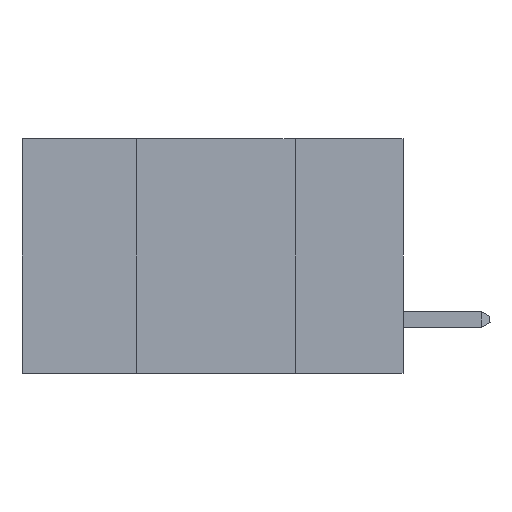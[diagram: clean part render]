
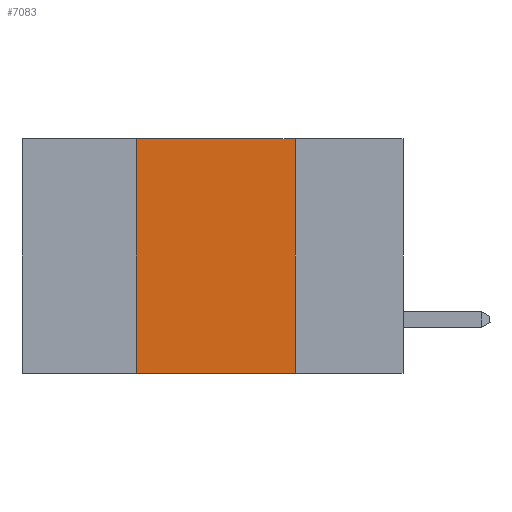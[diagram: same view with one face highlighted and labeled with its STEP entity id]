
A CAD part, left-side view. The second image highlights one B-rep face of the part: STEP entity #7083.
In plain terms, the highlighted planar face has unit normal (-1, 0, 0).
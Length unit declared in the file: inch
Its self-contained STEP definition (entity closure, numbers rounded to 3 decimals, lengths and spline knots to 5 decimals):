
#1003 = VERTEX_POINT ( 'NONE', #19001 ) ;
#2471 = EDGE_CURVE ( 'NONE', #4461, #5090, #20373, .T. ) ;
#3396 = EDGE_LOOP ( 'NONE', ( #16093, #5084, #22104, #19474 ) ) ;
#3500 = FACE_OUTER_BOUND ( 'NONE', #3396, .T. ) ;
#4435 = VECTOR ( 'NONE', #12951, 39.37008 ) ;
#4461 = VERTEX_POINT ( 'NONE', #22385 ) ;
#4968 = CARTESIAN_POINT ( 'NONE',  ( 0., 0.6, 0. ) ) ;
#5084 = ORIENTED_EDGE ( 'NONE', *, *, #2471, .F. ) ;
#5090 = VERTEX_POINT ( 'NONE', #24746 ) ;
#5324 = DIRECTION ( 'NONE',  ( 1., 0., 0. ) ) ;
#5408 = DIRECTION ( 'NONE',  ( 0., 0., -1. ) ) ;
#5662 = AXIS2_PLACEMENT_3D ( 'NONE', #4968, #5324, #5408 ) ;
#6020 = EDGE_CURVE ( 'NONE', #5090, #12776, #22463, .T. ) ;
#6211 = EDGE_CURVE ( 'NONE', #1003, #4461, #20874, .T. ) ;
#7083 = ADVANCED_FACE ( 'NONE', ( #3500 ), #17095, .F. ) ;
#7440 = CARTESIAN_POINT ( 'NONE',  ( 0., 0.42, 0. ) ) ;
#8737 = CARTESIAN_POINT ( 'NONE',  ( 0., 0.6, 0. ) ) ;
#11873 = CARTESIAN_POINT ( 'NONE',  ( 0., 0.6, -0.37 ) ) ;
#12776 = VERTEX_POINT ( 'NONE', #23280 ) ;
#12951 = DIRECTION ( 'NONE',  ( 0., 0., -1. ) ) ;
#13142 = CARTESIAN_POINT ( 'NONE',  ( 0., 0.17, 0. ) ) ;
#13583 = DIRECTION ( 'NONE',  ( 0., 0., 1. ) ) ;
#15518 = VECTOR ( 'NONE', #13583, 39.37008 ) ;
#15964 = VECTOR ( 'NONE', #23156, 39.37008 ) ;
#16093 = ORIENTED_EDGE ( 'NONE', *, *, #6020, .F. ) ;
#17095 = PLANE ( 'NONE',  #5662 ) ;
#19001 = CARTESIAN_POINT ( 'NONE',  ( 0., 0.42, -0.37 ) ) ;
#19474 = ORIENTED_EDGE ( 'NONE', *, *, #21866, .T. ) ;
#20373 = LINE ( 'NONE', #8737, #15964 ) ;
#20478 = LINE ( 'NONE', #11873, #22094 ) ;
#20874 = LINE ( 'NONE', #7440, #15518 ) ;
#21866 = EDGE_CURVE ( 'NONE', #1003, #12776, #20478, .T. ) ;
#22094 = VECTOR ( 'NONE', #25983, 39.37008 ) ;
#22104 = ORIENTED_EDGE ( 'NONE', *, *, #6211, .F. ) ;
#22385 = CARTESIAN_POINT ( 'NONE',  ( 0., 0.42, 0. ) ) ;
#22463 = LINE ( 'NONE', #13142, #4435 ) ;
#23156 = DIRECTION ( 'NONE',  ( 0., -1., 0. ) ) ;
#23280 = CARTESIAN_POINT ( 'NONE',  ( 0., 0.17, -0.37 ) ) ;
#24746 = CARTESIAN_POINT ( 'NONE',  ( 0., 0.17, 0. ) ) ;
#25983 = DIRECTION ( 'NONE',  ( 0., -1., 0. ) ) ;
